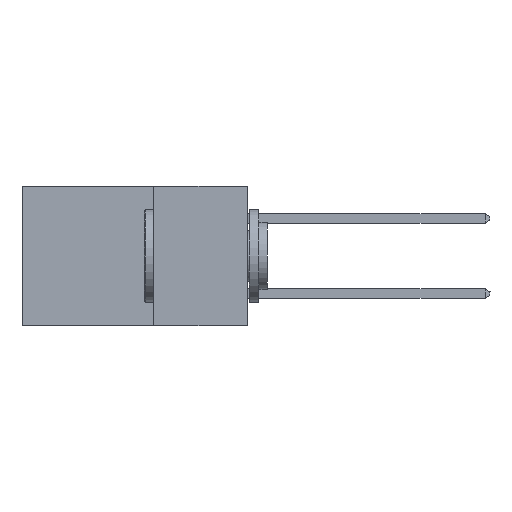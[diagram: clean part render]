
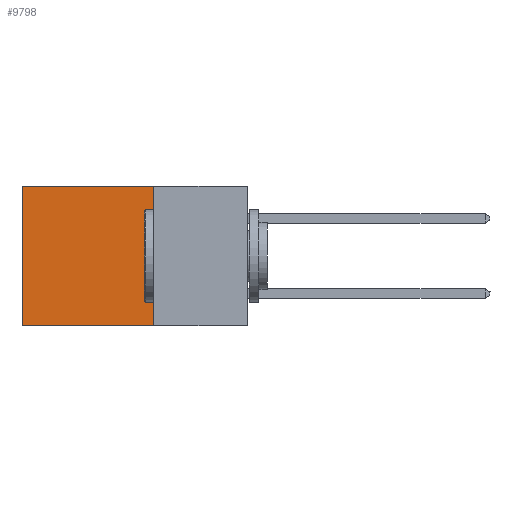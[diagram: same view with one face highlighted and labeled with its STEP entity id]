
A CAD part, left-side view. The second image highlights one B-rep face of the part: STEP entity #9798.
In plain terms, the highlighted planar face has unit normal (-1, 0, 0).
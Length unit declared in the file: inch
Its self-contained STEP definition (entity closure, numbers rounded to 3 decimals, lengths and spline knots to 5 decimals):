
#287 = CARTESIAN_POINT ( 'NONE',  ( 0.298, 0.6, 0. ) ) ;
#2025 = CARTESIAN_POINT ( 'NONE',  ( 0.298, 0.25, 0. ) ) ;
#2046 = CARTESIAN_POINT ( 'NONE',  ( 0.298, 0.25, -0.37 ) ) ;
#2113 = LINE ( 'NONE', #12160, #11447 ) ;
#2733 = FACE_OUTER_BOUND ( 'NONE', #4891, .T. ) ;
#3087 = LINE ( 'NONE', #16506, #12743 ) ;
#4891 = EDGE_LOOP ( 'NONE', ( #8468, #10393, #13272, #18203 ) ) ;
#5259 = CARTESIAN_POINT ( 'NONE',  ( 0.298, 0.6, 0. ) ) ;
#5293 = AXIS2_PLACEMENT_3D ( 'NONE', #21717, #12231, #8096 ) ;
#6445 = CARTESIAN_POINT ( 'NONE',  ( 0.298, 0.6, -0.37 ) ) ;
#7893 = DIRECTION ( 'NONE',  ( 0., 0., -1. ) ) ;
#8096 = DIRECTION ( 'NONE',  ( 0., 0., -1. ) ) ;
#8198 = VECTOR ( 'NONE', #8920, 39.37008 ) ;
#8226 = VERTEX_POINT ( 'NONE', #2025 ) ;
#8355 = DIRECTION ( 'NONE',  ( 0., 1., 0. ) ) ;
#8468 = ORIENTED_EDGE ( 'NONE', *, *, #21290, .T. ) ;
#8920 = DIRECTION ( 'NONE',  ( 0., 0., -1. ) ) ;
#9798 = ADVANCED_FACE ( 'NONE', ( #2733 ), #14015, .F. ) ;
#10393 = ORIENTED_EDGE ( 'NONE', *, *, #14885, .F. ) ;
#11447 = VECTOR ( 'NONE', #8355, 39.37008 ) ;
#12160 = CARTESIAN_POINT ( 'NONE',  ( 0.298, 0.25, 0. ) ) ;
#12231 = DIRECTION ( 'NONE',  ( 1., 0., 0. ) ) ;
#12647 = CARTESIAN_POINT ( 'NONE',  ( 0.298, 0.25, 0. ) ) ;
#12743 = VECTOR ( 'NONE', #20445, 39.37008 ) ;
#13272 = ORIENTED_EDGE ( 'NONE', *, *, #22345, .F. ) ;
#14015 = PLANE ( 'NONE',  #5293 ) ;
#14885 = EDGE_CURVE ( 'NONE', #16722, #24042, #3087, .T. ) ;
#15216 = VECTOR ( 'NONE', #7893, 39.37008 ) ;
#16482 = EDGE_CURVE ( 'NONE', #8226, #24471, #2113, .T. ) ;
#16506 = CARTESIAN_POINT ( 'NONE',  ( 0.298, 0.25, -0.37 ) ) ;
#16722 = VERTEX_POINT ( 'NONE', #2046 ) ;
#17850 = LINE ( 'NONE', #12647, #8198 ) ;
#18203 = ORIENTED_EDGE ( 'NONE', *, *, #16482, .T. ) ;
#20309 = LINE ( 'NONE', #287, #15216 ) ;
#20445 = DIRECTION ( 'NONE',  ( 0., 1., 0. ) ) ;
#21290 = EDGE_CURVE ( 'NONE', #24471, #24042, #20309, .T. ) ;
#21717 = CARTESIAN_POINT ( 'NONE',  ( 0.298, 0.25, 0. ) ) ;
#22345 = EDGE_CURVE ( 'NONE', #8226, #16722, #17850, .T. ) ;
#24042 = VERTEX_POINT ( 'NONE', #6445 ) ;
#24471 = VERTEX_POINT ( 'NONE', #5259 ) ;
